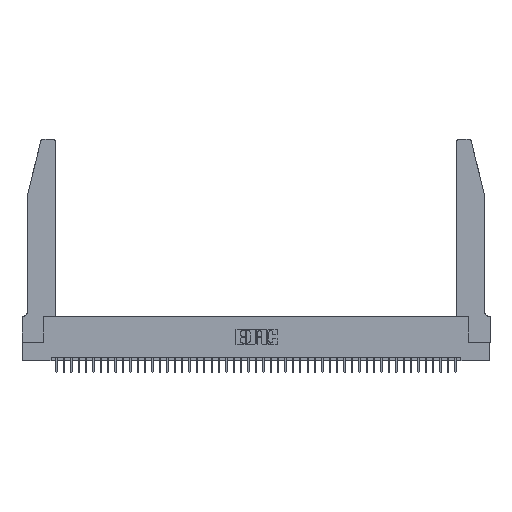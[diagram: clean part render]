
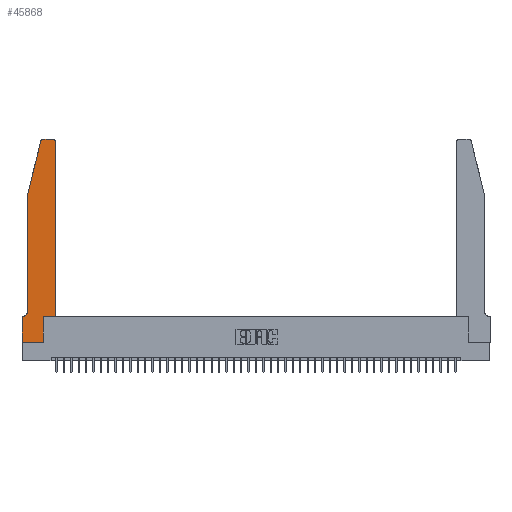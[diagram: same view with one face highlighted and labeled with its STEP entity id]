
A CAD part, top view. The second image highlights one B-rep face of the part: STEP entity #45868.
In plain terms, the highlighted planar face has unit normal (0, 0, 1).
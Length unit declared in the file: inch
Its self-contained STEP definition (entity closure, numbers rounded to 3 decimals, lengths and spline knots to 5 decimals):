
#208 = VERTEX_POINT ( 'NONE', #34202 ) ;
#1086 = VERTEX_POINT ( 'NONE', #28988 ) ;
#1119 = LINE ( 'NONE', #32747, #7178 ) ;
#1194 = VECTOR ( 'NONE', #34854, 39.37008 ) ;
#1799 = ORIENTED_EDGE ( 'NONE', *, *, #23564, .T. ) ;
#2820 = EDGE_CURVE ( 'NONE', #1086, #12180, #7908, .T. ) ;
#3814 = CARTESIAN_POINT ( 'NONE',  ( 0., 0.35, 0.37 ) ) ;
#3961 = ORIENTED_EDGE ( 'NONE', *, *, #26188, .T. ) ;
#4207 = CARTESIAN_POINT ( 'NONE',  ( 0., 0., 0.37 ) ) ;
#4231 = PLANE ( 'NONE',  #41288 ) ;
#4286 = CIRCLE ( 'NONE', #32224, 0.03 ) ;
#4721 = VECTOR ( 'NONE', #44467, 39.37008 ) ;
#5202 = CARTESIAN_POINT ( 'NONE',  ( 0.4505, 0.35, 0.37 ) ) ;
#5434 = FACE_OUTER_BOUND ( 'NONE', #6824, .T. ) ;
#5546 = VECTOR ( 'NONE', #9350, 39.37008 ) ;
#5726 = CARTESIAN_POINT ( 'NONE',  ( 0.4505, 0.35, 0.37 ) ) ;
#5788 = CIRCLE ( 'NONE', #6778, 0.07 ) ;
#5953 = VECTOR ( 'NONE', #43769, 39.37008 ) ;
#6295 = ORIENTED_EDGE ( 'NONE', *, *, #10370, .T. ) ;
#6778 = AXIS2_PLACEMENT_3D ( 'NONE', #31319, #9769, #34902 ) ;
#6824 = EDGE_LOOP ( 'NONE', ( #3961, #1799, #40444, #43772, #15920, #19334, #42677, #46020, #22152, #6295, #14298, #27212 ) ) ;
#7178 = VECTOR ( 'NONE', #25590, 39.37008 ) ;
#7652 = CARTESIAN_POINT ( 'NONE',  ( 0.284, 2.72, 0.37 ) ) ;
#7701 = LINE ( 'NONE', #13579, #24668 ) ;
#7908 = LINE ( 'NONE', #40433, #45967 ) ;
#8132 = EDGE_CURVE ( 'NONE', #21256, #23951, #25145, .T. ) ;
#9350 = DIRECTION ( 'NONE',  ( 0., 1., 0. ) ) ;
#9769 = DIRECTION ( 'NONE',  ( 0., 0., -1. ) ) ;
#10370 = EDGE_CURVE ( 'NONE', #20576, #26476, #21655, .T. ) ;
#10416 = VECTOR ( 'NONE', #15113, 39.37008 ) ;
#11117 = CARTESIAN_POINT ( 'NONE',  ( 0.2865, 0.35, 0.37 ) ) ;
#11330 = DIRECTION ( 'NONE',  ( 1., 0., 0. ) ) ;
#11410 = CARTESIAN_POINT ( 'NONE',  ( 0.4205, 2.72, 0.37 ) ) ;
#11493 = DIRECTION ( 'NONE',  ( 0., 0., 1. ) ) ;
#11591 = LINE ( 'NONE', #4207, #10416 ) ;
#11939 = CARTESIAN_POINT ( 'NONE',  ( 0.0755, 2., 0.37 ) ) ;
#12180 = VERTEX_POINT ( 'NONE', #11939 ) ;
#12616 = EDGE_CURVE ( 'NONE', #32303, #17107, #44891, .T. ) ;
#13579 = CARTESIAN_POINT ( 'NONE',  ( 0.0755, 2., 0.37 ) ) ;
#13618 = EDGE_CURVE ( 'NONE', #208, #21256, #14139, .T. ) ;
#13689 = EDGE_CURVE ( 'NONE', #21279, #20576, #39246, .T. ) ;
#14139 = LINE ( 'NONE', #30829, #41486 ) ;
#14298 = ORIENTED_EDGE ( 'NONE', *, *, #37290, .T. ) ;
#15062 = DIRECTION ( 'NONE',  ( 1., 0., 0. ) ) ;
#15113 = DIRECTION ( 'NONE',  ( 1., 0., 0. ) ) ;
#15920 = ORIENTED_EDGE ( 'NONE', *, *, #19316, .T. ) ;
#16448 = EDGE_CURVE ( 'NONE', #23951, #21279, #11591, .T. ) ;
#17107 = VERTEX_POINT ( 'NONE', #29329 ) ;
#19132 = DIRECTION ( 'NONE',  ( -0.239, -0.971, 0. ) ) ;
#19316 = EDGE_CURVE ( 'NONE', #29012, #208, #5788, .T. ) ;
#19334 = ORIENTED_EDGE ( 'NONE', *, *, #13618, .T. ) ;
#20576 = VERTEX_POINT ( 'NONE', #11117 ) ;
#21256 = VERTEX_POINT ( 'NONE', #3814 ) ;
#21279 = VERTEX_POINT ( 'NONE', #32561 ) ;
#21655 = LINE ( 'NONE', #5202, #4721 ) ;
#22152 = ORIENTED_EDGE ( 'NONE', *, *, #13689, .T. ) ;
#23564 = EDGE_CURVE ( 'NONE', #23849, #1086, #4286, .T. ) ;
#23849 = VERTEX_POINT ( 'NONE', #27189 ) ;
#23951 = VERTEX_POINT ( 'NONE', #45470 ) ;
#24668 = VECTOR ( 'NONE', #38534, 39.37008 ) ;
#24760 = CARTESIAN_POINT ( 'NONE',  ( 0.0755, 0.42, 0.37 ) ) ;
#25145 = LINE ( 'NONE', #26089, #5953 ) ;
#25590 = DIRECTION ( 'NONE',  ( -1., 0., 0. ) ) ;
#25857 = LINE ( 'NONE', #5726, #5546 ) ;
#26089 = CARTESIAN_POINT ( 'NONE',  ( 0., 0., 0.37 ) ) ;
#26188 = EDGE_CURVE ( 'NONE', #17107, #23849, #1119, .T. ) ;
#26224 = CARTESIAN_POINT ( 'NONE',  ( 0.4505, 2.72, 0.37 ) ) ;
#26476 = VERTEX_POINT ( 'NONE', #29175 ) ;
#27189 = CARTESIAN_POINT ( 'NONE',  ( 0.284, 2.75, 0.37 ) ) ;
#27212 = ORIENTED_EDGE ( 'NONE', *, *, #12616, .T. ) ;
#27367 = DIRECTION ( 'NONE',  ( -1., 0., 0. ) ) ;
#28988 = CARTESIAN_POINT ( 'NONE',  ( 0.25487, 2.72718, 0.37 ) ) ;
#29012 = VERTEX_POINT ( 'NONE', #24760 ) ;
#29175 = CARTESIAN_POINT ( 'NONE',  ( 0.4505, 0.35, 0.37 ) ) ;
#29329 = CARTESIAN_POINT ( 'NONE',  ( 0.4205, 2.75, 0.37 ) ) ;
#30829 = CARTESIAN_POINT ( 'NONE',  ( 0.0755, 0.35, 0.37 ) ) ;
#31319 = CARTESIAN_POINT ( 'NONE',  ( 0.0055, 0.42, 0.37 ) ) ;
#32224 = AXIS2_PLACEMENT_3D ( 'NONE', #7652, #32821, #11330 ) ;
#32303 = VERTEX_POINT ( 'NONE', #26224 ) ;
#32561 = CARTESIAN_POINT ( 'NONE',  ( 0.2865, 0., 0.37 ) ) ;
#32747 = CARTESIAN_POINT ( 'NONE',  ( 0.2605, 2.75, 0.37 ) ) ;
#32821 = DIRECTION ( 'NONE',  ( 0., 0., 1. ) ) ;
#32976 = CARTESIAN_POINT ( 'NONE',  ( 0., 0.35, 0.37 ) ) ;
#34202 = CARTESIAN_POINT ( 'NONE',  ( 0.0055, 0.35, 0.37 ) ) ;
#34854 = DIRECTION ( 'NONE',  ( 0., 1., 0. ) ) ;
#34902 = DIRECTION ( 'NONE',  ( -1., 0., 0. ) ) ;
#36485 = DIRECTION ( 'NONE',  ( 0., 0., 1. ) ) ;
#36554 = DIRECTION ( 'NONE',  ( 1., 0., 0. ) ) ;
#37290 = EDGE_CURVE ( 'NONE', #26476, #32303, #25857, .T. ) ;
#37592 = AXIS2_PLACEMENT_3D ( 'NONE', #11410, #36485, #15062 ) ;
#38383 = CARTESIAN_POINT ( 'NONE',  ( 0.2865, 0.35, 0.37 ) ) ;
#38534 = DIRECTION ( 'NONE',  ( 0., -1., 0. ) ) ;
#39246 = LINE ( 'NONE', #38383, #1194 ) ;
#40433 = CARTESIAN_POINT ( 'NONE',  ( 0.0755, 2., 0.37 ) ) ;
#40444 = ORIENTED_EDGE ( 'NONE', *, *, #2820, .T. ) ;
#41288 = AXIS2_PLACEMENT_3D ( 'NONE', #32976, #11493, #36554 ) ;
#41486 = VECTOR ( 'NONE', #27367, 39.37008 ) ;
#42677 = ORIENTED_EDGE ( 'NONE', *, *, #8132, .T. ) ;
#43357 = EDGE_CURVE ( 'NONE', #12180, #29012, #7701, .T. ) ;
#43769 = DIRECTION ( 'NONE',  ( 0., -1., 0. ) ) ;
#43772 = ORIENTED_EDGE ( 'NONE', *, *, #43357, .T. ) ;
#44467 = DIRECTION ( 'NONE',  ( 1., 0., 0. ) ) ;
#44891 = CIRCLE ( 'NONE', #37592, 0.03 ) ;
#45470 = CARTESIAN_POINT ( 'NONE',  ( 0., 0., 0.37 ) ) ;
#45868 = ADVANCED_FACE ( 'NONE', ( #5434 ), #4231, .T. ) ;
#45967 = VECTOR ( 'NONE', #19132, 39.37008 ) ;
#46020 = ORIENTED_EDGE ( 'NONE', *, *, #16448, .T. ) ;
